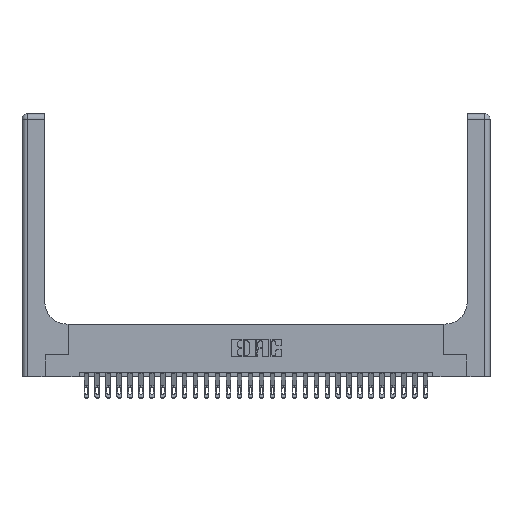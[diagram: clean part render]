
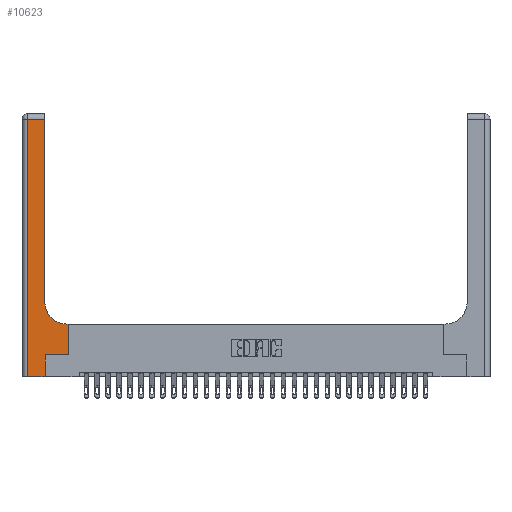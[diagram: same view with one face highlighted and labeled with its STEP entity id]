
A CAD part, top view. The second image highlights one B-rep face of the part: STEP entity #10623.
In plain terms, the highlighted planar face has unit normal (0, 0, 1).
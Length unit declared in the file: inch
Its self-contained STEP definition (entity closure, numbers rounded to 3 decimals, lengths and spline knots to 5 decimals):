
#12 = ORIENTED_EDGE ( 'NONE', *, *, #18353, .T. ) ;
#253 = ORIENTED_EDGE ( 'NONE', *, *, #21869, .T. ) ;
#643 = VERTEX_POINT ( 'NONE', #24083 ) ;
#680 = AXIS2_PLACEMENT_3D ( 'NONE', #24469, #17910, #2508 ) ;
#1065 = CARTESIAN_POINT ( 'NONE',  ( 0.06, 2.94, 0.37 ) ) ;
#1735 = VECTOR ( 'NONE', #4443, 39.37008 ) ;
#1975 = CARTESIAN_POINT ( 'NONE',  ( 0.265, 0., 0.37 ) ) ;
#2462 = CARTESIAN_POINT ( 'NONE',  ( 0.26, 3., 0.37 ) ) ;
#2508 = DIRECTION ( 'NONE',  ( -1., 0., 0. ) ) ;
#2524 = CARTESIAN_POINT ( 'NONE',  ( 0.26, 0.85, 0.37 ) ) ;
#3201 = DIRECTION ( 'NONE',  ( 1., 0., 0. ) ) ;
#3442 = EDGE_CURVE ( 'NONE', #643, #17283, #4513, .T. ) ;
#4159 = LINE ( 'NONE', #8449, #1735 ) ;
#4443 = DIRECTION ( 'NONE',  ( 0., -1., 0. ) ) ;
#4513 = LINE ( 'NONE', #6120, #24232 ) ;
#5134 = CARTESIAN_POINT ( 'NONE',  ( 0.26, 2.94, 0.37 ) ) ;
#5199 = ORIENTED_EDGE ( 'NONE', *, *, #26294, .T. ) ;
#6120 = CARTESIAN_POINT ( 'NONE',  ( 0.265, 0.25, 0.37 ) ) ;
#6968 = DIRECTION ( 'NONE',  ( 0., 1., 0. ) ) ;
#7195 = FACE_OUTER_BOUND ( 'NONE', #8323, .T. ) ;
#7203 = EDGE_CURVE ( 'NONE', #7458, #18432, #12404, .T. ) ;
#7303 = VERTEX_POINT ( 'NONE', #2524 ) ;
#7458 = VERTEX_POINT ( 'NONE', #13939 ) ;
#8262 = VECTOR ( 'NONE', #6968, 39.37008 ) ;
#8323 = EDGE_LOOP ( 'NONE', ( #253, #15382, #5199, #10347, #12, #16095, #22414, #21459, #17945 ) ) ;
#8449 = CARTESIAN_POINT ( 'NONE',  ( 0.06, 3., 0.37 ) ) ;
#8607 = VERTEX_POINT ( 'NONE', #1975 ) ;
#9439 = VERTEX_POINT ( 'NONE', #20455 ) ;
#10347 = ORIENTED_EDGE ( 'NONE', *, *, #17978, .T. ) ;
#10418 = DIRECTION ( 'NONE',  ( -1., 0., 0. ) ) ;
#10623 = ADVANCED_FACE ( 'NONE', ( #7195 ), #22172, .F. ) ;
#10728 = VERTEX_POINT ( 'NONE', #1065 ) ;
#10731 = CARTESIAN_POINT ( 'NONE',  ( 0.265, 0., 0.37 ) ) ;
#11640 = DIRECTION ( 'NONE',  ( 1., 0., 0. ) ) ;
#12404 = LINE ( 'NONE', #21080, #12801 ) ;
#12791 = LINE ( 'NONE', #21466, #17927 ) ;
#12801 = VECTOR ( 'NONE', #10418, 39.37008 ) ;
#12878 = EDGE_CURVE ( 'NONE', #18432, #7303, #27695, .T. ) ;
#13735 = LINE ( 'NONE', #2462, #25787 ) ;
#13939 = CARTESIAN_POINT ( 'NONE',  ( 0.528, 0.6, 0.37 ) ) ;
#14249 = CARTESIAN_POINT ( 'NONE',  ( 0.528, 0.25, 0.37 ) ) ;
#14555 = DIRECTION ( 'NONE',  ( 1., 0., 0. ) ) ;
#15088 = VERTEX_POINT ( 'NONE', #5134 ) ;
#15382 = ORIENTED_EDGE ( 'NONE', *, *, #25649, .T. ) ;
#15770 = CARTESIAN_POINT ( 'NONE',  ( 0., 2.94, 0.37 ) ) ;
#16051 = LINE ( 'NONE', #15770, #24932 ) ;
#16095 = ORIENTED_EDGE ( 'NONE', *, *, #3442, .T. ) ;
#17283 = VERTEX_POINT ( 'NONE', #14249 ) ;
#17910 = DIRECTION ( 'NONE',  ( 0., 0., -1. ) ) ;
#17927 = VECTOR ( 'NONE', #11640, 39.37008 ) ;
#17945 = ORIENTED_EDGE ( 'NONE', *, *, #12878, .T. ) ;
#17978 = EDGE_CURVE ( 'NONE', #9439, #8607, #12791, .T. ) ;
#18090 = EDGE_CURVE ( 'NONE', #17283, #7458, #22580, .T. ) ;
#18353 = EDGE_CURVE ( 'NONE', #8607, #643, #26521, .T. ) ;
#18432 = VERTEX_POINT ( 'NONE', #20240 ) ;
#20240 = CARTESIAN_POINT ( 'NONE',  ( 0.51, 0.6, 0.37 ) ) ;
#20445 = CARTESIAN_POINT ( 'NONE',  ( 0.528, 0.25, 0.37 ) ) ;
#20455 = CARTESIAN_POINT ( 'NONE',  ( 0.06, 0., 0.37 ) ) ;
#20670 = VECTOR ( 'NONE', #22300, 39.37008 ) ;
#21080 = CARTESIAN_POINT ( 'NONE',  ( 0.26, 0.6, 0.37 ) ) ;
#21459 = ORIENTED_EDGE ( 'NONE', *, *, #7203, .T. ) ;
#21466 = CARTESIAN_POINT ( 'NONE',  ( 0., 0., 0.37 ) ) ;
#21795 = DIRECTION ( 'NONE',  ( 0., 0., -1. ) ) ;
#21869 = EDGE_CURVE ( 'NONE', #7303, #15088, #13735, .T. ) ;
#22172 = PLANE ( 'NONE',  #680 ) ;
#22300 = DIRECTION ( 'NONE',  ( 0., 1., 0. ) ) ;
#22414 = ORIENTED_EDGE ( 'NONE', *, *, #18090, .T. ) ;
#22580 = LINE ( 'NONE', #20445, #20670 ) ;
#22603 = DIRECTION ( 'NONE',  ( -1., 0., 0. ) ) ;
#22727 = CARTESIAN_POINT ( 'NONE',  ( 0.51, 0.85, 0.37 ) ) ;
#24083 = CARTESIAN_POINT ( 'NONE',  ( 0.265, 0.25, 0.37 ) ) ;
#24232 = VECTOR ( 'NONE', #14555, 39.37008 ) ;
#24469 = CARTESIAN_POINT ( 'NONE',  ( 0., 3., 0.37 ) ) ;
#24932 = VECTOR ( 'NONE', #22603, 39.37008 ) ;
#25649 = EDGE_CURVE ( 'NONE', #15088, #10728, #16051, .T. ) ;
#25787 = VECTOR ( 'NONE', #26554, 39.37008 ) ;
#26294 = EDGE_CURVE ( 'NONE', #10728, #9439, #4159, .T. ) ;
#26318 = AXIS2_PLACEMENT_3D ( 'NONE', #22727, #21795, #3201 ) ;
#26521 = LINE ( 'NONE', #10731, #8262 ) ;
#26554 = DIRECTION ( 'NONE',  ( 0., 1., 0. ) ) ;
#27695 = CIRCLE ( 'NONE', #26318, 0.25 ) ;
